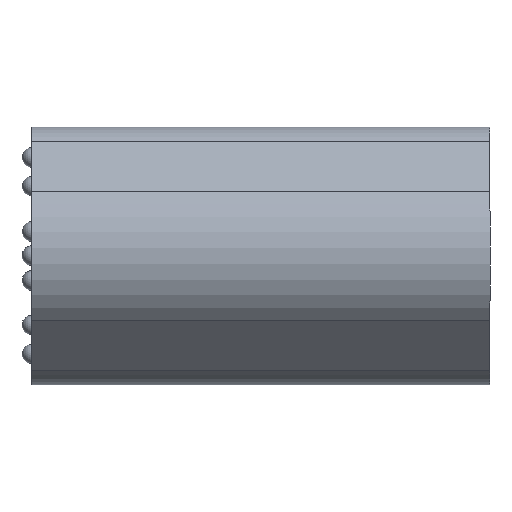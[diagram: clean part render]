
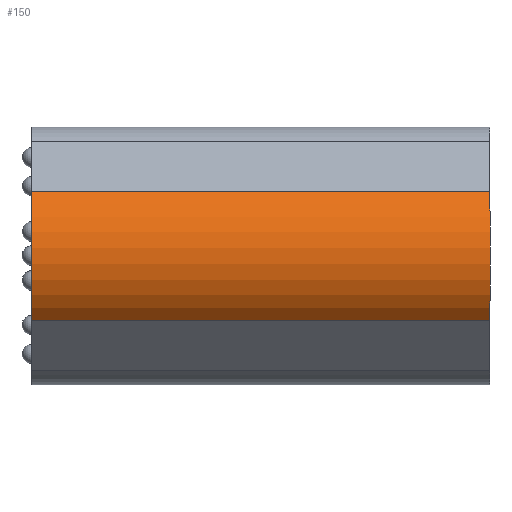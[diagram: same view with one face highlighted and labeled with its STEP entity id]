
A CAD part, left-side view. The second image highlights one B-rep face of the part: STEP entity #150.
In plain terms, the highlighted cylindrical face has radius 18.575 mm (diameter 37.15 mm), a partial arc.
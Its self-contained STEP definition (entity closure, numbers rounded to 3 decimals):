
#41 = EDGE_CURVE ( 'NONE', #1268, #2009, #1905, .T. ) ;
#150 = ADVANCED_FACE ( 'NONE', ( #1820 ), #1794, .T. ) ;
#405 = DIRECTION ( 'NONE',  ( 0., -1., 0. ) ) ;
#411 = DIRECTION ( 'NONE',  ( 0., 0., 1. ) ) ;
#434 = CARTESIAN_POINT ( 'NONE',  ( -193.405, 153.844, 4.547 ) ) ;
#448 = CARTESIAN_POINT ( 'NONE',  ( -206.54, 74.373, -8.587 ) ) ;
#454 = CARTESIAN_POINT ( 'NONE',  ( -206.54, -231.033, 17.682 ) ) ;
#510 = DIRECTION ( 'NONE',  ( 0., -1., 0. ) ) ;
#526 = EDGE_LOOP ( 'NONE', ( #1623, #1550, #1734, #1588 ) ) ;
#811 = DIRECTION ( 'NONE',  ( 0., 1., 0. ) ) ;
#819 = CARTESIAN_POINT ( 'NONE',  ( -206.54, 153.844, -8.587 ) ) ;
#822 = CARTESIAN_POINT ( 'NONE',  ( -206.54, 74.373, 17.682 ) ) ;
#837 = VECTOR ( 'NONE', #1315, 1000. ) ;
#840 = LINE ( 'NONE', #819, #837 ) ;
#890 = CIRCLE ( 'NONE', #1543, 18.575 ) ;
#945 = CIRCLE ( 'NONE', #1150, 18.575 ) ;
#990 = DIRECTION ( 'NONE',  ( 0., 1., 0. ) ) ;
#1150 = AXIS2_PLACEMENT_3D ( 'NONE', #1863, #990, #1998 ) ;
#1177 = VERTEX_POINT ( 'NONE', #448 ) ;
#1268 = VERTEX_POINT ( 'NONE', #822 ) ;
#1315 = DIRECTION ( 'NONE',  ( 0., -1., 0. ) ) ;
#1318 = CARTESIAN_POINT ( 'NONE',  ( -206.54, -18.876, -8.587 ) ) ;
#1343 = EDGE_CURVE ( 'NONE', #1177, #1268, #945, .T. ) ;
#1543 = AXIS2_PLACEMENT_3D ( 'NONE', #1713, #811, #1846 ) ;
#1550 = ORIENTED_EDGE ( 'NONE', *, *, #1631, .T. ) ;
#1588 = ORIENTED_EDGE ( 'NONE', *, *, #1343, .F. ) ;
#1623 = ORIENTED_EDGE ( 'NONE', *, *, #1792, .T. ) ;
#1631 = EDGE_CURVE ( 'NONE', #1901, #2009, #890, .T. ) ;
#1713 = CARTESIAN_POINT ( 'NONE',  ( -193.405, -18.876, 4.547 ) ) ;
#1734 = ORIENTED_EDGE ( 'NONE', *, *, #41, .F. ) ;
#1749 = AXIS2_PLACEMENT_3D ( 'NONE', #434, #405, #411 ) ;
#1792 = EDGE_CURVE ( 'NONE', #1177, #1901, #840, .T. ) ;
#1794 = CYLINDRICAL_SURFACE ( 'NONE', #1749, 18.575 ) ;
#1820 = FACE_OUTER_BOUND ( 'NONE', #526, .T. ) ;
#1846 = DIRECTION ( 'NONE',  ( 0., 0., 1. ) ) ;
#1863 = CARTESIAN_POINT ( 'NONE',  ( -193.405, 74.373, 4.547 ) ) ;
#1870 = CARTESIAN_POINT ( 'NONE',  ( -206.54, -18.876, 17.682 ) ) ;
#1899 = VECTOR ( 'NONE', #510, 1000. ) ;
#1901 = VERTEX_POINT ( 'NONE', #1318 ) ;
#1905 = LINE ( 'NONE', #454, #1899 ) ;
#1998 = DIRECTION ( 'NONE',  ( 0., 0., 1. ) ) ;
#2009 = VERTEX_POINT ( 'NONE', #1870 ) ;
